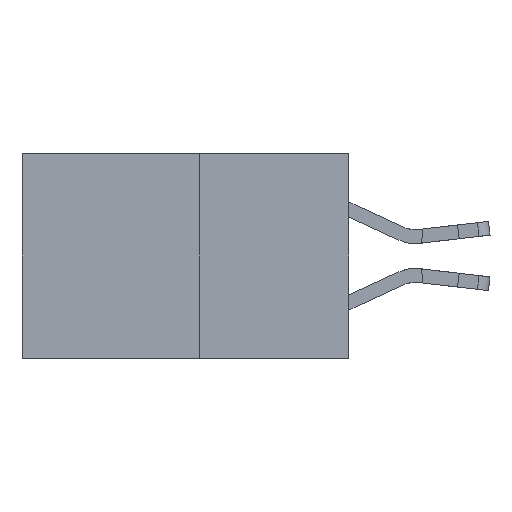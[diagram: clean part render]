
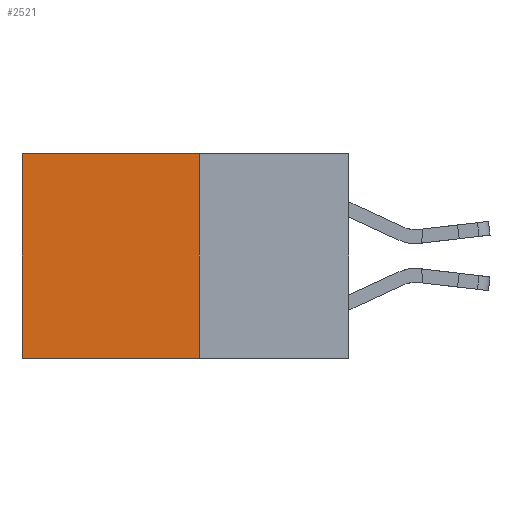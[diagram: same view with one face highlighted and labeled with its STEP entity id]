
A CAD part, left-side view. The second image highlights one B-rep face of the part: STEP entity #2521.
In plain terms, the highlighted planar face has unit normal (-1, 0, 0).
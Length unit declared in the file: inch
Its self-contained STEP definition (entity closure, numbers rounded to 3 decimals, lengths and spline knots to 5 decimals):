
#81 = LINE ( 'NONE', #5537, #12254 ) ;
#755 = EDGE_CURVE ( 'NONE', #9065, #3701, #81, .T. ) ;
#1051 = LINE ( 'NONE', #2147, #10452 ) ;
#1857 = EDGE_LOOP ( 'NONE', ( #9568, #4403, #11756, #3359 ) ) ;
#2004 = CARTESIAN_POINT ( 'NONE',  ( 0.277, 0.27, 0. ) ) ;
#2147 = CARTESIAN_POINT ( 'NONE',  ( 0.277, 0.27, -0.37 ) ) ;
#2521 = ADVANCED_FACE ( 'NONE', ( #7813 ), #4700, .F. ) ;
#3344 = LINE ( 'NONE', #6580, #3717 ) ;
#3359 = ORIENTED_EDGE ( 'NONE', *, *, #7184, .T. ) ;
#3493 = VERTEX_POINT ( 'NONE', #2004 ) ;
#3701 = VERTEX_POINT ( 'NONE', #9003 ) ;
#3717 = VECTOR ( 'NONE', #13524, 39.37008 ) ;
#4303 = EDGE_CURVE ( 'NONE', #3493, #4771, #3344, .T. ) ;
#4403 = ORIENTED_EDGE ( 'NONE', *, *, #10469, .F. ) ;
#4700 = PLANE ( 'NONE',  #14392 ) ;
#4771 = VERTEX_POINT ( 'NONE', #10855 ) ;
#5077 = CARTESIAN_POINT ( 'NONE',  ( 0.277, 0.59, 0. ) ) ;
#5537 = CARTESIAN_POINT ( 'NONE',  ( 0.277, 0.59, -0.37 ) ) ;
#6580 = CARTESIAN_POINT ( 'NONE',  ( 0.277, 0.27, -0.37 ) ) ;
#7184 = EDGE_CURVE ( 'NONE', #3493, #9065, #12540, .T. ) ;
#7642 = DIRECTION ( 'NONE',  ( 0., 1., 0. ) ) ;
#7813 = FACE_OUTER_BOUND ( 'NONE', #1857, .T. ) ;
#9003 = CARTESIAN_POINT ( 'NONE',  ( 0.277, 0.59, -0.37 ) ) ;
#9065 = VERTEX_POINT ( 'NONE', #5077 ) ;
#9568 = ORIENTED_EDGE ( 'NONE', *, *, #755, .T. ) ;
#9977 = DIRECTION ( 'NONE',  ( 1., 0., 0. ) ) ;
#10079 = DIRECTION ( 'NONE',  ( 0., 0., -1. ) ) ;
#10383 = DIRECTION ( 'NONE',  ( 0., 1., 0. ) ) ;
#10452 = VECTOR ( 'NONE', #10383, 39.37008 ) ;
#10469 = EDGE_CURVE ( 'NONE', #4771, #3701, #1051, .T. ) ;
#10855 = CARTESIAN_POINT ( 'NONE',  ( 0.277, 0.27, -0.37 ) ) ;
#11756 = ORIENTED_EDGE ( 'NONE', *, *, #4303, .F. ) ;
#12190 = VECTOR ( 'NONE', #7642, 39.37008 ) ;
#12254 = VECTOR ( 'NONE', #10079, 39.37008 ) ;
#12540 = LINE ( 'NONE', #14476, #12190 ) ;
#12790 = DIRECTION ( 'NONE',  ( 0., 0., -1. ) ) ;
#13109 = CARTESIAN_POINT ( 'NONE',  ( 0.277, 0.27, -0.37 ) ) ;
#13524 = DIRECTION ( 'NONE',  ( 0., 0., -1. ) ) ;
#14392 = AXIS2_PLACEMENT_3D ( 'NONE', #13109, #9977, #12790 ) ;
#14476 = CARTESIAN_POINT ( 'NONE',  ( 0.277, 0.27, 0. ) ) ;
